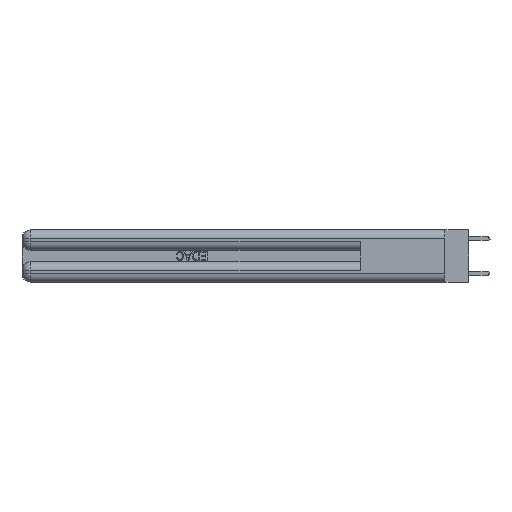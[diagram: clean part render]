
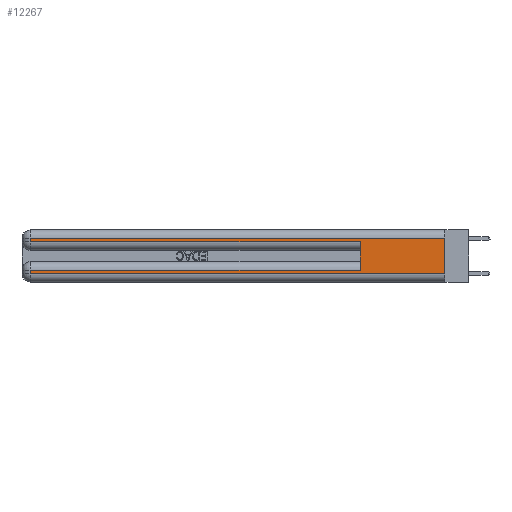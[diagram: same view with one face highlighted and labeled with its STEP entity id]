
A CAD part, left-side view. The second image highlights one B-rep face of the part: STEP entity #12267.
In plain terms, the highlighted planar face has unit normal (-1, 0, 0).
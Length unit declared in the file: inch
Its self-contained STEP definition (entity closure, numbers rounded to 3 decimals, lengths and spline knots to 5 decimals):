
#350 = DIRECTION ( 'NONE',  ( 0., 0., 1. ) ) ;
#866 = CARTESIAN_POINT ( 'NONE',  ( 0., 2.94, 0.06 ) ) ;
#2181 = VERTEX_POINT ( 'NONE', #4629 ) ;
#2793 = LINE ( 'NONE', #5370, #21003 ) ;
#2934 = ORIENTED_EDGE ( 'NONE', *, *, #27085, .T. ) ;
#3457 = CARTESIAN_POINT ( 'NONE',  ( 0., 0., 0.085 ) ) ;
#3466 = EDGE_CURVE ( 'NONE', #2181, #10506, #4338, .T. ) ;
#4338 = LINE ( 'NONE', #23507, #5079 ) ;
#4629 = CARTESIAN_POINT ( 'NONE',  ( 0., 2.94, 0.285 ) ) ;
#5079 = VECTOR ( 'NONE', #9423, 39.37008 ) ;
#5370 = CARTESIAN_POINT ( 'NONE',  ( 0., 0., 0.06 ) ) ;
#5662 = CARTESIAN_POINT ( 'NONE',  ( 0., 0.6, 0.085 ) ) ;
#5866 = DIRECTION ( 'NONE',  ( 0., 1., 0. ) ) ;
#6098 = DIRECTION ( 'NONE',  ( 0., 0., -1. ) ) ;
#6293 = EDGE_LOOP ( 'NONE', ( #28745, #16664, #14110, #18920, #25151, #14135, #2934, #12301 ) ) ;
#6420 = LINE ( 'NONE', #18178, #12766 ) ;
#6633 = DIRECTION ( 'NONE',  ( 0., 0., -1. ) ) ;
#7547 = VERTEX_POINT ( 'NONE', #29925 ) ;
#8368 = FACE_OUTER_BOUND ( 'NONE', #6293, .T. ) ;
#8433 = CARTESIAN_POINT ( 'NONE',  ( 0., 0., 0.37 ) ) ;
#9209 = DIRECTION ( 'NONE',  ( 0., 1., 0. ) ) ;
#9319 = VERTEX_POINT ( 'NONE', #27648 ) ;
#9423 = DIRECTION ( 'NONE',  ( 0., -1., 0. ) ) ;
#10506 = VERTEX_POINT ( 'NONE', #25636 ) ;
#10801 = EDGE_CURVE ( 'NONE', #15298, #9319, #2793, .T. ) ;
#10942 = EDGE_CURVE ( 'NONE', #20466, #7547, #17290, .T. ) ;
#11093 = DIRECTION ( 'NONE',  ( 0., 0., -1. ) ) ;
#11577 = LINE ( 'NONE', #21566, #16338 ) ;
#11748 = VECTOR ( 'NONE', #6633, 39.37008 ) ;
#12267 = ADVANCED_FACE ( 'NONE', ( #8368 ), #29612, .F. ) ;
#12301 = ORIENTED_EDGE ( 'NONE', *, *, #10801, .T. ) ;
#12766 = VECTOR ( 'NONE', #11093, 39.37008 ) ;
#12776 = AXIS2_PLACEMENT_3D ( 'NONE', #8433, #20284, #6098 ) ;
#13825 = EDGE_CURVE ( 'NONE', #13962, #27610, #17876, .T. ) ;
#13962 = VERTEX_POINT ( 'NONE', #28690 ) ;
#14110 = ORIENTED_EDGE ( 'NONE', *, *, #15480, .T. ) ;
#14135 = ORIENTED_EDGE ( 'NONE', *, *, #10942, .T. ) ;
#14697 = CARTESIAN_POINT ( 'NONE',  ( 0., 0.6, 0.145 ) ) ;
#15298 = VERTEX_POINT ( 'NONE', #866 ) ;
#15480 = EDGE_CURVE ( 'NONE', #27610, #2181, #6420, .T. ) ;
#16338 = VECTOR ( 'NONE', #23923, 39.37008 ) ;
#16664 = ORIENTED_EDGE ( 'NONE', *, *, #13825, .T. ) ;
#17288 = VECTOR ( 'NONE', #350, 39.37008 ) ;
#17290 = LINE ( 'NONE', #3457, #29034 ) ;
#17876 = LINE ( 'NONE', #20939, #24112 ) ;
#18178 = CARTESIAN_POINT ( 'NONE',  ( 0., 2.94, 0.37 ) ) ;
#18920 = ORIENTED_EDGE ( 'NONE', *, *, #3466, .T. ) ;
#20284 = DIRECTION ( 'NONE',  ( 1., 0., 0. ) ) ;
#20466 = VERTEX_POINT ( 'NONE', #5662 ) ;
#20939 = CARTESIAN_POINT ( 'NONE',  ( 0., 0., 0.31 ) ) ;
#21003 = VECTOR ( 'NONE', #26631, 39.37008 ) ;
#21566 = CARTESIAN_POINT ( 'NONE',  ( 0., 0., 0.37 ) ) ;
#23507 = CARTESIAN_POINT ( 'NONE',  ( 0., 0., 0.285 ) ) ;
#23923 = DIRECTION ( 'NONE',  ( 0., 0., -1. ) ) ;
#24112 = VECTOR ( 'NONE', #9209, 39.37008 ) ;
#24220 = LINE ( 'NONE', #25392, #11748 ) ;
#25151 = ORIENTED_EDGE ( 'NONE', *, *, #25507, .F. ) ;
#25392 = CARTESIAN_POINT ( 'NONE',  ( 0., 2.94, 0.37 ) ) ;
#25507 = EDGE_CURVE ( 'NONE', #20466, #10506, #29784, .T. ) ;
#25636 = CARTESIAN_POINT ( 'NONE',  ( 0., 0.6, 0.285 ) ) ;
#26631 = DIRECTION ( 'NONE',  ( 0., -1., 0. ) ) ;
#27085 = EDGE_CURVE ( 'NONE', #7547, #15298, #24220, .T. ) ;
#27610 = VERTEX_POINT ( 'NONE', #27701 ) ;
#27648 = CARTESIAN_POINT ( 'NONE',  ( 0., 0., 0.06 ) ) ;
#27701 = CARTESIAN_POINT ( 'NONE',  ( 0., 2.94, 0.31 ) ) ;
#28690 = CARTESIAN_POINT ( 'NONE',  ( 0., 0., 0.31 ) ) ;
#28745 = ORIENTED_EDGE ( 'NONE', *, *, #30519, .F. ) ;
#29034 = VECTOR ( 'NONE', #5866, 39.37008 ) ;
#29612 = PLANE ( 'NONE',  #12776 ) ;
#29784 = LINE ( 'NONE', #14697, #17288 ) ;
#29925 = CARTESIAN_POINT ( 'NONE',  ( 0., 2.94, 0.085 ) ) ;
#30519 = EDGE_CURVE ( 'NONE', #13962, #9319, #11577, .T. ) ;
